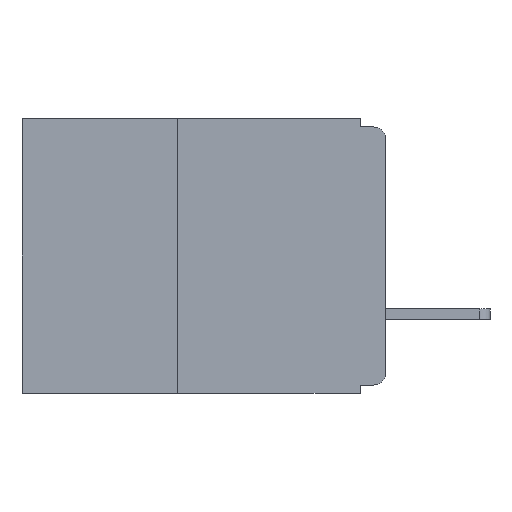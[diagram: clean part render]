
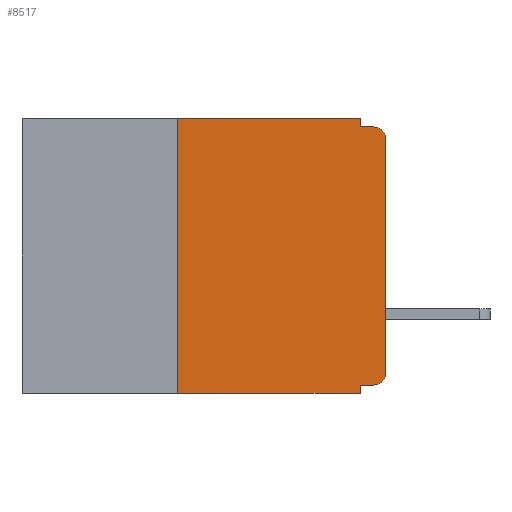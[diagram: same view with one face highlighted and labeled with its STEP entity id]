
A CAD part, left-side view. The second image highlights one B-rep face of the part: STEP entity #8517.
In plain terms, the highlighted planar face has unit normal (-1, 0, 0).
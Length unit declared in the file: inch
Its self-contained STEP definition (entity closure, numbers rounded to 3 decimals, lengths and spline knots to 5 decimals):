
#486 = CARTESIAN_POINT ( 'NONE',  ( 0., 0., -0.305 ) ) ;
#753 = ORIENTED_EDGE ( 'NONE', *, *, #2711, .F. ) ;
#765 = AXIS2_PLACEMENT_3D ( 'NONE', #3522, #13905, #4992 ) ;
#1295 = EDGE_CURVE ( 'NONE', #4659, #15026, #7391, .T. ) ;
#1311 = VECTOR ( 'NONE', #15923, 39.37008 ) ;
#1384 = AXIS2_PLACEMENT_3D ( 'NONE', #7077, #17507, #8560 ) ;
#1509 = CARTESIAN_POINT ( 'NONE',  ( 0., 0., -0.01 ) ) ;
#1526 = VECTOR ( 'NONE', #17742, 39.37008 ) ;
#1594 = CARTESIAN_POINT ( 'NONE',  ( 0., 0., -0.025 ) ) ;
#1799 = LINE ( 'NONE', #16371, #1311 ) ;
#2180 = DIRECTION ( 'NONE',  ( 0., 0., 1. ) ) ;
#2351 = EDGE_CURVE ( 'NONE', #5652, #18303, #7823, .T. ) ;
#2357 = CARTESIAN_POINT ( 'NONE',  ( 0., 0., -0.32 ) ) ;
#2400 = CARTESIAN_POINT ( 'NONE',  ( 0., 0.031, -0.33 ) ) ;
#2693 = DIRECTION ( 'NONE',  ( 0., 0., -1. ) ) ;
#2711 = EDGE_CURVE ( 'NONE', #7965, #13823, #1799, .T. ) ;
#2976 = VECTOR ( 'NONE', #15465, 39.37008 ) ;
#2986 = VECTOR ( 'NONE', #14915, 39.37008 ) ;
#3174 = EDGE_LOOP ( 'NONE', ( #14733, #3798, #7733, #15667, #753, #4708, #17080, #9609, #10068, #14041 ) ) ;
#3271 = CARTESIAN_POINT ( 'NONE',  ( 0., 0.25, -0.33 ) ) ;
#3388 = VERTEX_POINT ( 'NONE', #17894 ) ;
#3440 = FACE_OUTER_BOUND ( 'NONE', #3174, .T. ) ;
#3522 = CARTESIAN_POINT ( 'NONE',  ( 0., 0.015, -0.025 ) ) ;
#3798 = ORIENTED_EDGE ( 'NONE', *, *, #17186, .T. ) ;
#3905 = DIRECTION ( 'NONE',  ( 0., 0., -1. ) ) ;
#3985 = DIRECTION ( 'NONE',  ( 0., 0., -1. ) ) ;
#4094 = PLANE ( 'NONE',  #1384 ) ;
#4659 = VERTEX_POINT ( 'NONE', #3271 ) ;
#4708 = ORIENTED_EDGE ( 'NONE', *, *, #9267, .F. ) ;
#4992 = DIRECTION ( 'NONE',  ( 0., 0., -1. ) ) ;
#5186 = EDGE_CURVE ( 'NONE', #12306, #5652, #7020, .T. ) ;
#5652 = VERTEX_POINT ( 'NONE', #486 ) ;
#5873 = LINE ( 'NONE', #2400, #13300 ) ;
#5947 = LINE ( 'NONE', #11751, #1526 ) ;
#7020 = CIRCLE ( 'NONE', #17193, 0.015 ) ;
#7077 = CARTESIAN_POINT ( 'NONE',  ( 0., 0.437, 0. ) ) ;
#7391 = LINE ( 'NONE', #18114, #2976 ) ;
#7733 = ORIENTED_EDGE ( 'NONE', *, *, #8064, .F. ) ;
#7796 = LINE ( 'NONE', #11628, #15280 ) ;
#7823 = LINE ( 'NONE', #17685, #11358 ) ;
#7921 = CARTESIAN_POINT ( 'NONE',  ( 0., 0.031, 0. ) ) ;
#7965 = VERTEX_POINT ( 'NONE', #16148 ) ;
#8064 = EDGE_CURVE ( 'NONE', #3388, #10403, #14857, .T. ) ;
#8517 = ADVANCED_FACE ( 'NONE', ( #3440 ), #4094, .F. ) ;
#8560 = DIRECTION ( 'NONE',  ( 0., 0., -1. ) ) ;
#9267 = EDGE_CURVE ( 'NONE', #4659, #7965, #5947, .T. ) ;
#9609 = ORIENTED_EDGE ( 'NONE', *, *, #11649, .F. ) ;
#10068 = ORIENTED_EDGE ( 'NONE', *, *, #12800, .F. ) ;
#10403 = VERTEX_POINT ( 'NONE', #18821 ) ;
#11096 = CIRCLE ( 'NONE', #765, 0.015 ) ;
#11286 = DIRECTION ( 'NONE',  ( -1., 0., 0. ) ) ;
#11354 = CARTESIAN_POINT ( 'NONE',  ( 0., 0.015, -0.305 ) ) ;
#11358 = VECTOR ( 'NONE', #2180, 39.37008 ) ;
#11558 = CARTESIAN_POINT ( 'NONE',  ( 0., 0.015, -0.32 ) ) ;
#11628 = CARTESIAN_POINT ( 'NONE',  ( 0., 0.031, 0. ) ) ;
#11649 = EDGE_CURVE ( 'NONE', #14282, #15026, #5873, .T. ) ;
#11751 = CARTESIAN_POINT ( 'NONE',  ( 0., 0.25, -0.33 ) ) ;
#12030 = CARTESIAN_POINT ( 'NONE',  ( 0., 0.031, -0.32 ) ) ;
#12202 = CARTESIAN_POINT ( 'NONE',  ( 0., 0.031, -0.33 ) ) ;
#12306 = VERTEX_POINT ( 'NONE', #11558 ) ;
#12589 = LINE ( 'NONE', #2357, #13482 ) ;
#12754 = DIRECTION ( 'NONE',  ( 0., 1., 0. ) ) ;
#12800 = EDGE_CURVE ( 'NONE', #12306, #14282, #12589, .T. ) ;
#13300 = VECTOR ( 'NONE', #3905, 39.37008 ) ;
#13482 = VECTOR ( 'NONE', #12754, 39.37008 ) ;
#13823 = VERTEX_POINT ( 'NONE', #7921 ) ;
#13905 = DIRECTION ( 'NONE',  ( -1., 0., 0. ) ) ;
#14041 = ORIENTED_EDGE ( 'NONE', *, *, #5186, .T. ) ;
#14282 = VERTEX_POINT ( 'NONE', #12030 ) ;
#14733 = ORIENTED_EDGE ( 'NONE', *, *, #2351, .T. ) ;
#14857 = LINE ( 'NONE', #1509, #2986 ) ;
#14915 = DIRECTION ( 'NONE',  ( 0., -1., 0. ) ) ;
#15026 = VERTEX_POINT ( 'NONE', #12202 ) ;
#15280 = VECTOR ( 'NONE', #2693, 39.37008 ) ;
#15465 = DIRECTION ( 'NONE',  ( 0., -1., 0. ) ) ;
#15667 = ORIENTED_EDGE ( 'NONE', *, *, #16260, .F. ) ;
#15923 = DIRECTION ( 'NONE',  ( 0., -1., 0. ) ) ;
#16148 = CARTESIAN_POINT ( 'NONE',  ( 0., 0.25, 0. ) ) ;
#16260 = EDGE_CURVE ( 'NONE', #13823, #3388, #7796, .T. ) ;
#16371 = CARTESIAN_POINT ( 'NONE',  ( 0., 0.437, 0. ) ) ;
#17080 = ORIENTED_EDGE ( 'NONE', *, *, #1295, .T. ) ;
#17186 = EDGE_CURVE ( 'NONE', #18303, #10403, #11096, .T. ) ;
#17193 = AXIS2_PLACEMENT_3D ( 'NONE', #11354, #11286, #3985 ) ;
#17507 = DIRECTION ( 'NONE',  ( 1., 0., 0. ) ) ;
#17685 = CARTESIAN_POINT ( 'NONE',  ( 0., 0., 0. ) ) ;
#17742 = DIRECTION ( 'NONE',  ( 0., 0., 1. ) ) ;
#17894 = CARTESIAN_POINT ( 'NONE',  ( 0., 0.031, -0.01 ) ) ;
#18114 = CARTESIAN_POINT ( 'NONE',  ( 0., 0.437, -0.33 ) ) ;
#18303 = VERTEX_POINT ( 'NONE', #1594 ) ;
#18821 = CARTESIAN_POINT ( 'NONE',  ( 0., 0.015, -0.01 ) ) ;
